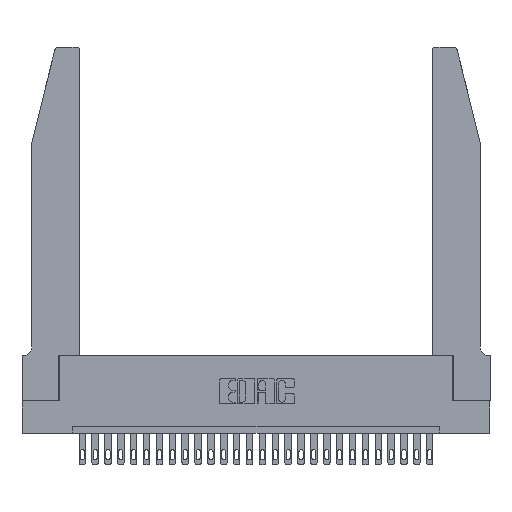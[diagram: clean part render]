
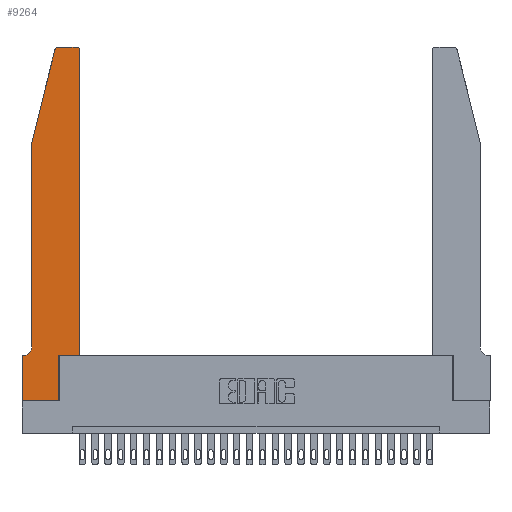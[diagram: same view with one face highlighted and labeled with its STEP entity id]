
A CAD part, top view. The second image highlights one B-rep face of the part: STEP entity #9264.
In plain terms, the highlighted planar face has unit normal (0, 0, 1).
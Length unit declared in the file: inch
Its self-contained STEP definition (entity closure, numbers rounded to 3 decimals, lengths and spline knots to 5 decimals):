
#91 = EDGE_LOOP ( 'NONE', ( #17648, #550, #8952, #10435, #9808, #10743, #23790, #739, #4917, #9137, #13713, #13113 ) ) ;
#114 = CIRCLE ( 'NONE', #6647, 0.03 ) ;
#324 = CIRCLE ( 'NONE', #14243, 0.03 ) ;
#550 = ORIENTED_EDGE ( 'NONE', *, *, #14897, .T. ) ;
#739 = ORIENTED_EDGE ( 'NONE', *, *, #10660, .T. ) ;
#1523 = LINE ( 'NONE', #11058, #17870 ) ;
#2449 = VECTOR ( 'NONE', #27401, 39.37008 ) ;
#2784 = CARTESIAN_POINT ( 'NONE',  ( 0., 0., 0.37 ) ) ;
#3064 = VERTEX_POINT ( 'NONE', #10378 ) ;
#3185 = CARTESIAN_POINT ( 'NONE',  ( 0.4505, 0.35, 0.37 ) ) ;
#3794 = VECTOR ( 'NONE', #6141, 39.37008 ) ;
#4740 = VERTEX_POINT ( 'NONE', #12944 ) ;
#4917 = ORIENTED_EDGE ( 'NONE', *, *, #8304, .T. ) ;
#5240 = CARTESIAN_POINT ( 'NONE',  ( 0.25487, 2.72718, 0.37 ) ) ;
#5409 = VECTOR ( 'NONE', #16658, 39.37008 ) ;
#5569 = VECTOR ( 'NONE', #18207, 39.37008 ) ;
#5578 = VERTEX_POINT ( 'NONE', #25022 ) ;
#5790 = PLANE ( 'NONE',  #27093 ) ;
#5814 = CARTESIAN_POINT ( 'NONE',  ( 0.4505, 0.35, 0.37 ) ) ;
#6141 = DIRECTION ( 'NONE',  ( -1., 0., 0. ) ) ;
#6189 = DIRECTION ( 'NONE',  ( 0., -1., 0. ) ) ;
#6247 = CARTESIAN_POINT ( 'NONE',  ( 0.4505, 0.35, 0.37 ) ) ;
#6328 = DIRECTION ( 'NONE',  ( -1., 0., 0. ) ) ;
#6515 = DIRECTION ( 'NONE',  ( 0., 0., 1. ) ) ;
#6647 = AXIS2_PLACEMENT_3D ( 'NONE', #16598, #18738, #22811 ) ;
#6738 = VERTEX_POINT ( 'NONE', #5240 ) ;
#7158 = CARTESIAN_POINT ( 'NONE',  ( 0.2865, 0.35, 0.37 ) ) ;
#7227 = LINE ( 'NONE', #15783, #5569 ) ;
#8304 = EDGE_CURVE ( 'NONE', #13148, #15208, #20485, .T. ) ;
#8392 = VERTEX_POINT ( 'NONE', #3185 ) ;
#8749 = LINE ( 'NONE', #27603, #18093 ) ;
#8754 = DIRECTION ( 'NONE',  ( -1., 0., 0. ) ) ;
#8952 = ORIENTED_EDGE ( 'NONE', *, *, #24407, .T. ) ;
#9137 = ORIENTED_EDGE ( 'NONE', *, *, #14386, .T. ) ;
#9264 = ADVANCED_FACE ( 'NONE', ( #26039 ), #5790, .T. ) ;
#9802 = DIRECTION ( 'NONE',  ( 1., 0., 0. ) ) ;
#9808 = ORIENTED_EDGE ( 'NONE', *, *, #27225, .T. ) ;
#10260 = CARTESIAN_POINT ( 'NONE',  ( 0.0055, 0.42, 0.37 ) ) ;
#10378 = CARTESIAN_POINT ( 'NONE',  ( 0.4205, 2.75, 0.37 ) ) ;
#10435 = ORIENTED_EDGE ( 'NONE', *, *, #10499, .T. ) ;
#10499 = EDGE_CURVE ( 'NONE', #26348, #23874, #19033, .T. ) ;
#10660 = EDGE_CURVE ( 'NONE', #5578, #13148, #20673, .T. ) ;
#10743 = ORIENTED_EDGE ( 'NONE', *, *, #14534, .T. ) ;
#11058 = CARTESIAN_POINT ( 'NONE',  ( 0.0755, 0.35, 0.37 ) ) ;
#11111 = LINE ( 'NONE', #21171, #3794 ) ;
#11883 = VERTEX_POINT ( 'NONE', #12199 ) ;
#11990 = DIRECTION ( 'NONE',  ( 0., 1., 0. ) ) ;
#12199 = CARTESIAN_POINT ( 'NONE',  ( 0., 0.35, 0.37 ) ) ;
#12409 = CARTESIAN_POINT ( 'NONE',  ( 0.0755, 2., 0.37 ) ) ;
#12657 = VECTOR ( 'NONE', #27079, 39.37008 ) ;
#12944 = CARTESIAN_POINT ( 'NONE',  ( 0.0055, 0.35, 0.37 ) ) ;
#12962 = VECTOR ( 'NONE', #21998, 39.37008 ) ;
#13113 = ORIENTED_EDGE ( 'NONE', *, *, #27497, .T. ) ;
#13148 = VERTEX_POINT ( 'NONE', #26494 ) ;
#13713 = ORIENTED_EDGE ( 'NONE', *, *, #15773, .T. ) ;
#14136 = EDGE_CURVE ( 'NONE', #3064, #21139, #11111, .T. ) ;
#14243 = AXIS2_PLACEMENT_3D ( 'NONE', #25610, #6515, #17177 ) ;
#14386 = EDGE_CURVE ( 'NONE', #15208, #8392, #22537, .T. ) ;
#14534 = EDGE_CURVE ( 'NONE', #4740, #11883, #1523, .T. ) ;
#14897 = EDGE_CURVE ( 'NONE', #21139, #6738, #114, .T. ) ;
#15208 = VERTEX_POINT ( 'NONE', #23737 ) ;
#15773 = EDGE_CURVE ( 'NONE', #8392, #22312, #16816, .T. ) ;
#15783 = CARTESIAN_POINT ( 'NONE',  ( 0.0755, 2., 0.37 ) ) ;
#16003 = CARTESIAN_POINT ( 'NONE',  ( 0.0755, 0.42, 0.37 ) ) ;
#16598 = CARTESIAN_POINT ( 'NONE',  ( 0.284, 2.72, 0.37 ) ) ;
#16658 = DIRECTION ( 'NONE',  ( 0., 1., 0. ) ) ;
#16816 = LINE ( 'NONE', #5814, #5409 ) ;
#17177 = DIRECTION ( 'NONE',  ( 1., 0., 0. ) ) ;
#17648 = ORIENTED_EDGE ( 'NONE', *, *, #14136, .T. ) ;
#17798 = VECTOR ( 'NONE', #11990, 39.37008 ) ;
#17870 = VECTOR ( 'NONE', #8754, 39.37008 ) ;
#18093 = VECTOR ( 'NONE', #6189, 39.37008 ) ;
#18207 = DIRECTION ( 'NONE',  ( -0.239, -0.971, 0. ) ) ;
#18738 = DIRECTION ( 'NONE',  ( 0., 0., 1. ) ) ;
#19033 = LINE ( 'NONE', #26777, #12657 ) ;
#20457 = CARTESIAN_POINT ( 'NONE',  ( 0., 0.35, 0.37 ) ) ;
#20485 = LINE ( 'NONE', #7158, #17798 ) ;
#20673 = LINE ( 'NONE', #2784, #12962 ) ;
#21139 = VERTEX_POINT ( 'NONE', #21925 ) ;
#21171 = CARTESIAN_POINT ( 'NONE',  ( 0.2605, 2.75, 0.37 ) ) ;
#21435 = CARTESIAN_POINT ( 'NONE',  ( 0.4505, 2.72, 0.37 ) ) ;
#21461 = EDGE_CURVE ( 'NONE', #11883, #5578, #8749, .T. ) ;
#21885 = AXIS2_PLACEMENT_3D ( 'NONE', #10260, #23395, #6328 ) ;
#21925 = CARTESIAN_POINT ( 'NONE',  ( 0.284, 2.75, 0.37 ) ) ;
#21998 = DIRECTION ( 'NONE',  ( 1., 0., 0. ) ) ;
#22312 = VERTEX_POINT ( 'NONE', #21435 ) ;
#22537 = LINE ( 'NONE', #6247, #2449 ) ;
#22584 = DIRECTION ( 'NONE',  ( 0., 0., 1. ) ) ;
#22811 = DIRECTION ( 'NONE',  ( 1., 0., 0. ) ) ;
#23395 = DIRECTION ( 'NONE',  ( 0., 0., -1. ) ) ;
#23737 = CARTESIAN_POINT ( 'NONE',  ( 0.2865, 0.35, 0.37 ) ) ;
#23790 = ORIENTED_EDGE ( 'NONE', *, *, #21461, .T. ) ;
#23874 = VERTEX_POINT ( 'NONE', #16003 ) ;
#24407 = EDGE_CURVE ( 'NONE', #6738, #26348, #7227, .T. ) ;
#25022 = CARTESIAN_POINT ( 'NONE',  ( 0., 0., 0.37 ) ) ;
#25610 = CARTESIAN_POINT ( 'NONE',  ( 0.4205, 2.72, 0.37 ) ) ;
#26039 = FACE_OUTER_BOUND ( 'NONE', #91, .T. ) ;
#26348 = VERTEX_POINT ( 'NONE', #12409 ) ;
#26494 = CARTESIAN_POINT ( 'NONE',  ( 0.2865, 0., 0.37 ) ) ;
#26777 = CARTESIAN_POINT ( 'NONE',  ( 0.0755, 2., 0.37 ) ) ;
#27079 = DIRECTION ( 'NONE',  ( 0., -1., 0. ) ) ;
#27093 = AXIS2_PLACEMENT_3D ( 'NONE', #20457, #22584, #9802 ) ;
#27225 = EDGE_CURVE ( 'NONE', #23874, #4740, #27436, .T. ) ;
#27401 = DIRECTION ( 'NONE',  ( 1., 0., 0. ) ) ;
#27436 = CIRCLE ( 'NONE', #21885, 0.07 ) ;
#27497 = EDGE_CURVE ( 'NONE', #22312, #3064, #324, .T. ) ;
#27603 = CARTESIAN_POINT ( 'NONE',  ( 0., 0., 0.37 ) ) ;
